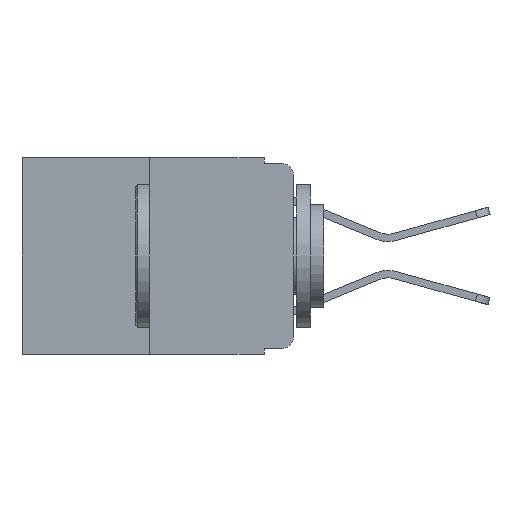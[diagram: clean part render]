
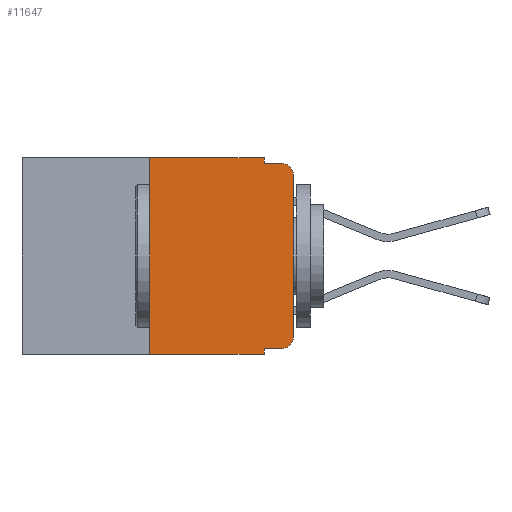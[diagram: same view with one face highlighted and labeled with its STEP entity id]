
A CAD part, left-side view. The second image highlights one B-rep face of the part: STEP entity #11647.
In plain terms, the highlighted planar face has unit normal (-1, 0, 0).
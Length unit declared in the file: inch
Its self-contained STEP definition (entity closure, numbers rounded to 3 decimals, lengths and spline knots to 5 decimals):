
#21 = CARTESIAN_POINT ( 'NONE',  ( 0., 0.02, -0.01 ) ) ;
#539 = VECTOR ( 'NONE', #17064, 39.37008 ) ;
#941 = CARTESIAN_POINT ( 'NONE',  ( 0., 0.473, 0. ) ) ;
#1194 = DIRECTION ( 'NONE',  ( -1., 0., 0. ) ) ;
#1690 = CARTESIAN_POINT ( 'NONE',  ( 0., 0., -0.03 ) ) ;
#1812 = CARTESIAN_POINT ( 'NONE',  ( 0., 0.051, -0.333 ) ) ;
#1857 = VERTEX_POINT ( 'NONE', #13146 ) ;
#2141 = VECTOR ( 'NONE', #21755, 39.37008 ) ;
#2810 = EDGE_CURVE ( 'NONE', #1857, #5369, #15796, .T. ) ;
#2816 = CARTESIAN_POINT ( 'NONE',  ( 0., 0.051, 0. ) ) ;
#3747 = VERTEX_POINT ( 'NONE', #9474 ) ;
#3966 = CARTESIAN_POINT ( 'NONE',  ( 0., 0.473, -0.343 ) ) ;
#4765 = LINE ( 'NONE', #5451, #17249 ) ;
#5158 = LINE ( 'NONE', #5202, #539 ) ;
#5202 = CARTESIAN_POINT ( 'NONE',  ( 0., 0.473, 0. ) ) ;
#5369 = VERTEX_POINT ( 'NONE', #15065 ) ;
#5451 = CARTESIAN_POINT ( 'NONE',  ( 0., 0., 0. ) ) ;
#5692 = DIRECTION ( 'NONE',  ( 0., -1., 0. ) ) ;
#5831 = VERTEX_POINT ( 'NONE', #21 ) ;
#5903 = ORIENTED_EDGE ( 'NONE', *, *, #18437, .F. ) ;
#5904 = AXIS2_PLACEMENT_3D ( 'NONE', #11427, #1194, #13116 ) ;
#6128 = LINE ( 'NONE', #9399, #14635 ) ;
#6236 = EDGE_CURVE ( 'NONE', #5369, #17526, #14203, .T. ) ;
#6562 = AXIS2_PLACEMENT_3D ( 'NONE', #941, #7927, #19757 ) ;
#7142 = DIRECTION ( 'NONE',  ( 0., 0., 1. ) ) ;
#7464 = ORIENTED_EDGE ( 'NONE', *, *, #14767, .T. ) ;
#7503 = EDGE_CURVE ( 'NONE', #17386, #5831, #11223, .T. ) ;
#7618 = CARTESIAN_POINT ( 'NONE',  ( 0., 0., -0.313 ) ) ;
#7756 = ORIENTED_EDGE ( 'NONE', *, *, #15055, .F. ) ;
#7927 = DIRECTION ( 'NONE',  ( 1., 0., 0. ) ) ;
#7929 = FACE_OUTER_BOUND ( 'NONE', #21763, .T. ) ;
#8410 = CARTESIAN_POINT ( 'NONE',  ( 0., 0.25, 0. ) ) ;
#8485 = LINE ( 'NONE', #2816, #17500 ) ;
#9399 = CARTESIAN_POINT ( 'NONE',  ( 0., 0.051, 0. ) ) ;
#9474 = CARTESIAN_POINT ( 'NONE',  ( 0., 0.25, -0.343 ) ) ;
#9776 = DIRECTION ( 'NONE',  ( -1., 0., 0. ) ) ;
#10106 = VERTEX_POINT ( 'NONE', #14110 ) ;
#10129 = DIRECTION ( 'NONE',  ( 0., 0., 1. ) ) ;
#10466 = VECTOR ( 'NONE', #10129, 39.37008 ) ;
#10558 = EDGE_CURVE ( 'NONE', #17226, #13688, #5158, .T. ) ;
#10980 = LINE ( 'NONE', #8410, #10466 ) ;
#11097 = DIRECTION ( 'NONE',  ( 0., 0., -1. ) ) ;
#11223 = LINE ( 'NONE', #16737, #2141 ) ;
#11224 = DIRECTION ( 'NONE',  ( 0., 0., -1. ) ) ;
#11305 = VECTOR ( 'NONE', #15495, 39.37008 ) ;
#11427 = CARTESIAN_POINT ( 'NONE',  ( 0., 0.02, -0.313 ) ) ;
#11647 = ADVANCED_FACE ( 'NONE', ( #7929 ), #16385, .F. ) ;
#12145 = CARTESIAN_POINT ( 'NONE',  ( 0., 0.051, 0. ) ) ;
#12492 = CIRCLE ( 'NONE', #18320, 0.02 ) ;
#12541 = ORIENTED_EDGE ( 'NONE', *, *, #20281, .F. ) ;
#13116 = DIRECTION ( 'NONE',  ( 0., 0., -1. ) ) ;
#13146 = CARTESIAN_POINT ( 'NONE',  ( 0., 0.051, -0.333 ) ) ;
#13562 = CARTESIAN_POINT ( 'NONE',  ( 0., 0.25, 0. ) ) ;
#13571 = ORIENTED_EDGE ( 'NONE', *, *, #7503, .F. ) ;
#13688 = VERTEX_POINT ( 'NONE', #12145 ) ;
#13783 = EDGE_CURVE ( 'NONE', #3747, #10106, #18955, .T. ) ;
#14007 = CARTESIAN_POINT ( 'NONE',  ( 0., 0.051, -0.01 ) ) ;
#14110 = CARTESIAN_POINT ( 'NONE',  ( 0., 0.051, -0.343 ) ) ;
#14203 = CIRCLE ( 'NONE', #5904, 0.02 ) ;
#14456 = ORIENTED_EDGE ( 'NONE', *, *, #6236, .T. ) ;
#14635 = VECTOR ( 'NONE', #11097, 39.37008 ) ;
#14767 = EDGE_CURVE ( 'NONE', #17526, #20597, #4765, .T. ) ;
#15055 = EDGE_CURVE ( 'NONE', #13688, #17386, #8485, .T. ) ;
#15065 = CARTESIAN_POINT ( 'NONE',  ( 0., 0.02, -0.333 ) ) ;
#15495 = DIRECTION ( 'NONE',  ( 0., -1., 0. ) ) ;
#15796 = LINE ( 'NONE', #1812, #11305 ) ;
#16385 = PLANE ( 'NONE',  #6562 ) ;
#16495 = ORIENTED_EDGE ( 'NONE', *, *, #20406, .T. ) ;
#16737 = CARTESIAN_POINT ( 'NONE',  ( 0., 0.051, -0.01 ) ) ;
#17064 = DIRECTION ( 'NONE',  ( 0., -1., 0. ) ) ;
#17226 = VERTEX_POINT ( 'NONE', #13562 ) ;
#17249 = VECTOR ( 'NONE', #7142, 39.37008 ) ;
#17386 = VERTEX_POINT ( 'NONE', #14007 ) ;
#17500 = VECTOR ( 'NONE', #11224, 39.37008 ) ;
#17526 = VERTEX_POINT ( 'NONE', #7618 ) ;
#18320 = AXIS2_PLACEMENT_3D ( 'NONE', #19872, #9776, #21543 ) ;
#18413 = VECTOR ( 'NONE', #5692, 39.37008 ) ;
#18437 = EDGE_CURVE ( 'NONE', #3747, #17226, #10980, .T. ) ;
#18662 = ORIENTED_EDGE ( 'NONE', *, *, #2810, .T. ) ;
#18955 = LINE ( 'NONE', #3966, #18413 ) ;
#19757 = DIRECTION ( 'NONE',  ( 0., 0., -1. ) ) ;
#19872 = CARTESIAN_POINT ( 'NONE',  ( 0., 0.02, -0.03 ) ) ;
#19941 = ORIENTED_EDGE ( 'NONE', *, *, #13783, .T. ) ;
#20281 = EDGE_CURVE ( 'NONE', #1857, #10106, #6128, .T. ) ;
#20406 = EDGE_CURVE ( 'NONE', #20597, #5831, #12492, .T. ) ;
#20597 = VERTEX_POINT ( 'NONE', #1690 ) ;
#21543 = DIRECTION ( 'NONE',  ( 0., 0., -1. ) ) ;
#21741 = ORIENTED_EDGE ( 'NONE', *, *, #10558, .F. ) ;
#21755 = DIRECTION ( 'NONE',  ( 0., -1., 0. ) ) ;
#21763 = EDGE_LOOP ( 'NONE', ( #7464, #16495, #13571, #7756, #21741, #5903, #19941, #12541, #18662, #14456 ) ) ;
